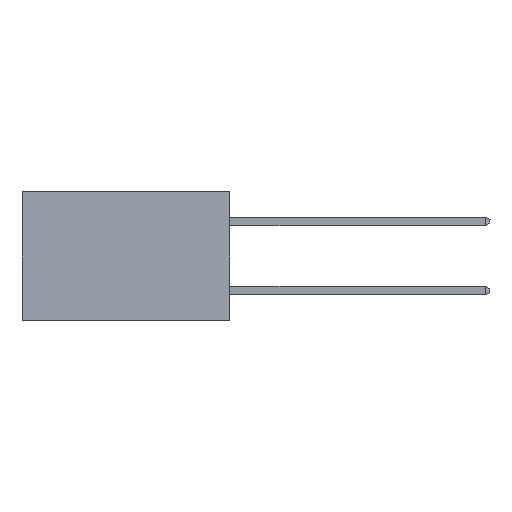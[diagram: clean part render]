
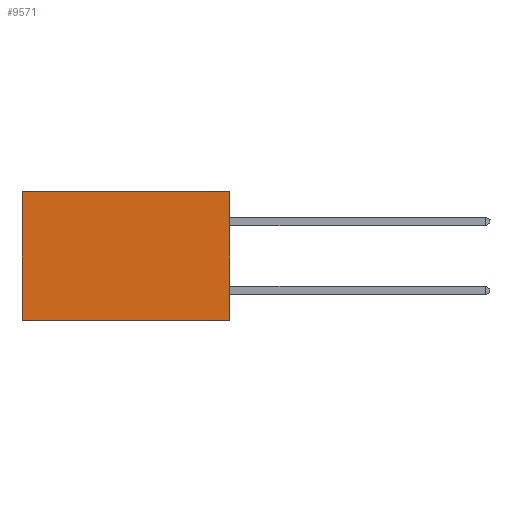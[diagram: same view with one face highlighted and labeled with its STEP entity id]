
A CAD part, left-side view. The second image highlights one B-rep face of the part: STEP entity #9571.
In plain terms, the highlighted planar face has unit normal (-1, 0, 0).
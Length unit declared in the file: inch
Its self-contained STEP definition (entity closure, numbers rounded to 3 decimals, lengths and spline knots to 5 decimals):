
#131 = CARTESIAN_POINT ( 'NONE',  ( 0.2615, 0., -0.37 ) ) ;
#344 = DIRECTION ( 'NONE',  ( 0., 1., 0. ) ) ;
#605 = ORIENTED_EDGE ( 'NONE', *, *, #4135, .T. ) ;
#643 = EDGE_CURVE ( 'NONE', #2085, #8864, #9602, .T. ) ;
#1688 = CARTESIAN_POINT ( 'NONE',  ( 0.2615, 0., -0.37 ) ) ;
#1797 = CARTESIAN_POINT ( 'NONE',  ( 0.2615, 0., -0.37 ) ) ;
#2085 = VERTEX_POINT ( 'NONE', #2973 ) ;
#2571 = ORIENTED_EDGE ( 'NONE', *, *, #643, .F. ) ;
#2698 = EDGE_LOOP ( 'NONE', ( #605, #7234, #2571, #9374 ) ) ;
#2811 = VERTEX_POINT ( 'NONE', #11090 ) ;
#2973 = CARTESIAN_POINT ( 'NONE',  ( 0.2615, 0., 0. ) ) ;
#4135 = EDGE_CURVE ( 'NONE', #2811, #4387, #8857, .T. ) ;
#4387 = VERTEX_POINT ( 'NONE', #6916 ) ;
#4491 = DIRECTION ( 'NONE',  ( 0., 1., 0. ) ) ;
#5495 = DIRECTION ( 'NONE',  ( 0., 0., -1. ) ) ;
#5995 = LINE ( 'NONE', #1688, #12472 ) ;
#6916 = CARTESIAN_POINT ( 'NONE',  ( 0.2615, 0.6, -0.37 ) ) ;
#7026 = VECTOR ( 'NONE', #344, 39.37008 ) ;
#7234 = ORIENTED_EDGE ( 'NONE', *, *, #9617, .F. ) ;
#8559 = AXIS2_PLACEMENT_3D ( 'NONE', #12636, #9747, #11143 ) ;
#8857 = LINE ( 'NONE', #11493, #14675 ) ;
#8864 = VERTEX_POINT ( 'NONE', #1797 ) ;
#8950 = DIRECTION ( 'NONE',  ( 0., 0., -1. ) ) ;
#9374 = ORIENTED_EDGE ( 'NONE', *, *, #16168, .T. ) ;
#9571 = ADVANCED_FACE ( 'NONE', ( #12375 ), #9931, .F. ) ;
#9602 = LINE ( 'NONE', #131, #14259 ) ;
#9617 = EDGE_CURVE ( 'NONE', #8864, #4387, #5995, .T. ) ;
#9747 = DIRECTION ( 'NONE',  ( 1., 0., 0. ) ) ;
#9931 = PLANE ( 'NONE',  #8559 ) ;
#11046 = CARTESIAN_POINT ( 'NONE',  ( 0.2615, 0., 0. ) ) ;
#11090 = CARTESIAN_POINT ( 'NONE',  ( 0.2615, 0.6, 0. ) ) ;
#11143 = DIRECTION ( 'NONE',  ( 0., 0., -1. ) ) ;
#11493 = CARTESIAN_POINT ( 'NONE',  ( 0.2615, 0.6, -0.37 ) ) ;
#12375 = FACE_OUTER_BOUND ( 'NONE', #2698, .T. ) ;
#12472 = VECTOR ( 'NONE', #4491, 39.37008 ) ;
#12636 = CARTESIAN_POINT ( 'NONE',  ( 0.2615, 0., -0.37 ) ) ;
#13495 = LINE ( 'NONE', #11046, #7026 ) ;
#14259 = VECTOR ( 'NONE', #5495, 39.37008 ) ;
#14675 = VECTOR ( 'NONE', #8950, 39.37008 ) ;
#16168 = EDGE_CURVE ( 'NONE', #2085, #2811, #13495, .T. ) ;
